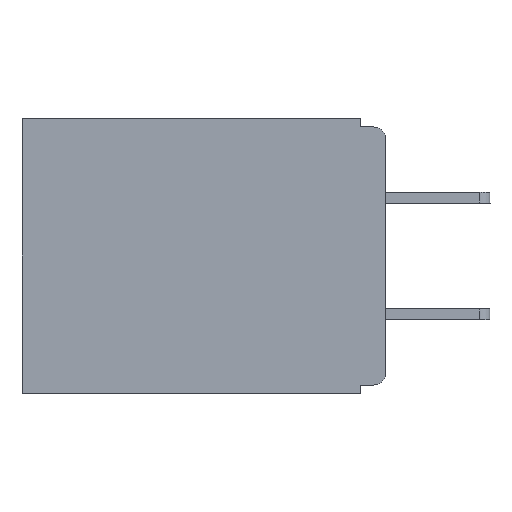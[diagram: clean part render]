
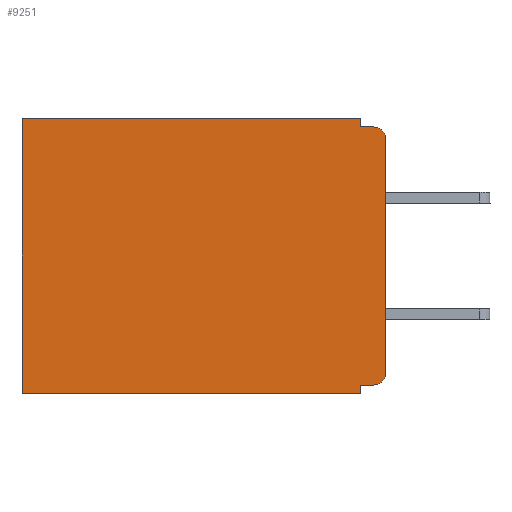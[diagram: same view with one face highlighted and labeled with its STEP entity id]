
A CAD part, left-side view. The second image highlights one B-rep face of the part: STEP entity #9251.
In plain terms, the highlighted planar face has unit normal (-1, 0, 0).
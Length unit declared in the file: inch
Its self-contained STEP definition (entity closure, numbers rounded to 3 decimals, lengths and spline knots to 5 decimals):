
#112 = CARTESIAN_POINT ( 'NONE',  ( 0.3, 0., -0.33 ) ) ;
#113 = ORIENTED_EDGE ( 'NONE', *, *, #10455, .T. ) ;
#322 = VECTOR ( 'NONE', #4174, 39.37008 ) ;
#392 = VERTEX_POINT ( 'NONE', #700 ) ;
#411 = ORIENTED_EDGE ( 'NONE', *, *, #10589, .T. ) ;
#700 = CARTESIAN_POINT ( 'NONE',  ( 0.3, 0.031, -0.01 ) ) ;
#881 = DIRECTION ( 'NONE',  ( 0., 0., -1. ) ) ;
#925 = VECTOR ( 'NONE', #10698, 39.37008 ) ;
#952 = LINE ( 'NONE', #10044, #9979 ) ;
#1090 = EDGE_CURVE ( 'NONE', #5036, #7505, #2635, .T. ) ;
#1230 = EDGE_CURVE ( 'NONE', #2956, #392, #1493, .T. ) ;
#1237 = VECTOR ( 'NONE', #881, 39.37008 ) ;
#1493 = LINE ( 'NONE', #9932, #1237 ) ;
#1507 = EDGE_LOOP ( 'NONE', ( #8773, #411, #9183, #10623, #9588, #2218, #10093, #7792, #8123, #113 ) ) ;
#1562 = DIRECTION ( 'NONE',  ( 0., 0., -1. ) ) ;
#1647 = CIRCLE ( 'NONE', #2615, 0.015 ) ;
#1676 = EDGE_CURVE ( 'NONE', #10653, #7437, #5539, .T. ) ;
#1992 = EDGE_CURVE ( 'NONE', #2956, #8823, #952, .T. ) ;
#2188 = VECTOR ( 'NONE', #4564, 39.37008 ) ;
#2218 = ORIENTED_EDGE ( 'NONE', *, *, #5886, .T. ) ;
#2301 = DIRECTION ( 'NONE',  ( -1., 0., 0. ) ) ;
#2525 = DIRECTION ( 'NONE',  ( 0., 0., -1. ) ) ;
#2615 = AXIS2_PLACEMENT_3D ( 'NONE', #8127, #2301, #7282 ) ;
#2635 = LINE ( 'NONE', #8255, #322 ) ;
#2956 = VERTEX_POINT ( 'NONE', #6523 ) ;
#3293 = EDGE_CURVE ( 'NONE', #392, #8702, #8289, .T. ) ;
#3481 = VERTEX_POINT ( 'NONE', #6968 ) ;
#3605 = VERTEX_POINT ( 'NONE', #6253 ) ;
#3878 = CARTESIAN_POINT ( 'NONE',  ( 0.3, 0.031, -0.33 ) ) ;
#4119 = DIRECTION ( 'NONE',  ( 0., 1., 0. ) ) ;
#4156 = EDGE_CURVE ( 'NONE', #7437, #3481, #9274, .T. ) ;
#4174 = DIRECTION ( 'NONE',  ( 0., 0., -1. ) ) ;
#4404 = CARTESIAN_POINT ( 'NONE',  ( 0.3, 0.437, 0. ) ) ;
#4564 = DIRECTION ( 'NONE',  ( 0., 1., 0. ) ) ;
#4778 = CARTESIAN_POINT ( 'NONE',  ( 0.3, 0., -0.025 ) ) ;
#4897 = VECTOR ( 'NONE', #4119, 39.37008 ) ;
#5036 = VERTEX_POINT ( 'NONE', #4778 ) ;
#5539 = LINE ( 'NONE', #3878, #9664 ) ;
#5593 = AXIS2_PLACEMENT_3D ( 'NONE', #9767, #8970, #1562 ) ;
#5886 = EDGE_CURVE ( 'NONE', #8823, #3481, #10051, .T. ) ;
#6253 = CARTESIAN_POINT ( 'NONE',  ( 0.3, 0.015, -0.32 ) ) ;
#6406 = DIRECTION ( 'NONE',  ( 0., 0., -1. ) ) ;
#6487 = LINE ( 'NONE', #8383, #4897 ) ;
#6523 = CARTESIAN_POINT ( 'NONE',  ( 0.3, 0.031, 0. ) ) ;
#6708 = PLANE ( 'NONE',  #6716 ) ;
#6716 = AXIS2_PLACEMENT_3D ( 'NONE', #112, #9090, #2525 ) ;
#6800 = DIRECTION ( 'NONE',  ( 0., 1., 0. ) ) ;
#6950 = CARTESIAN_POINT ( 'NONE',  ( 0.3, 0., -0.305 ) ) ;
#6968 = CARTESIAN_POINT ( 'NONE',  ( 0.3, 0.437, -0.33 ) ) ;
#7282 = DIRECTION ( 'NONE',  ( 0., 0., -1. ) ) ;
#7308 = CARTESIAN_POINT ( 'NONE',  ( 0.3, 0., -0.01 ) ) ;
#7437 = VERTEX_POINT ( 'NONE', #10022 ) ;
#7505 = VERTEX_POINT ( 'NONE', #6950 ) ;
#7650 = FACE_OUTER_BOUND ( 'NONE', #1507, .T. ) ;
#7792 = ORIENTED_EDGE ( 'NONE', *, *, #1676, .F. ) ;
#7889 = VECTOR ( 'NONE', #9708, 39.37008 ) ;
#8123 = ORIENTED_EDGE ( 'NONE', *, *, #8329, .F. ) ;
#8127 = CARTESIAN_POINT ( 'NONE',  ( 0.3, 0.015, -0.025 ) ) ;
#8255 = CARTESIAN_POINT ( 'NONE',  ( 0.3, 0., -0.33 ) ) ;
#8289 = LINE ( 'NONE', #7308, #925 ) ;
#8329 = EDGE_CURVE ( 'NONE', #3605, #10653, #6487, .T. ) ;
#8383 = CARTESIAN_POINT ( 'NONE',  ( 0.3, 0., -0.32 ) ) ;
#8702 = VERTEX_POINT ( 'NONE', #10594 ) ;
#8773 = ORIENTED_EDGE ( 'NONE', *, *, #1090, .F. ) ;
#8823 = VERTEX_POINT ( 'NONE', #4404 ) ;
#8970 = DIRECTION ( 'NONE',  ( -1., 0., 0. ) ) ;
#9090 = DIRECTION ( 'NONE',  ( 1., 0., 0. ) ) ;
#9183 = ORIENTED_EDGE ( 'NONE', *, *, #3293, .F. ) ;
#9251 = ADVANCED_FACE ( 'NONE', ( #7650 ), #6708, .F. ) ;
#9274 = LINE ( 'NONE', #9475, #2188 ) ;
#9475 = CARTESIAN_POINT ( 'NONE',  ( 0.3, 0., -0.33 ) ) ;
#9588 = ORIENTED_EDGE ( 'NONE', *, *, #1992, .T. ) ;
#9664 = VECTOR ( 'NONE', #6406, 39.37008 ) ;
#9708 = DIRECTION ( 'NONE',  ( 0., 0., -1. ) ) ;
#9726 = CARTESIAN_POINT ( 'NONE',  ( 0.3, 0.031, -0.32 ) ) ;
#9767 = CARTESIAN_POINT ( 'NONE',  ( 0.3, 0.015, -0.305 ) ) ;
#9893 = CIRCLE ( 'NONE', #5593, 0.015 ) ;
#9932 = CARTESIAN_POINT ( 'NONE',  ( 0.3, 0.031, 0. ) ) ;
#9979 = VECTOR ( 'NONE', #6800, 39.37008 ) ;
#10022 = CARTESIAN_POINT ( 'NONE',  ( 0.3, 0.031, -0.33 ) ) ;
#10044 = CARTESIAN_POINT ( 'NONE',  ( 0.3, 0., 0. ) ) ;
#10051 = LINE ( 'NONE', #10435, #7889 ) ;
#10093 = ORIENTED_EDGE ( 'NONE', *, *, #4156, .F. ) ;
#10435 = CARTESIAN_POINT ( 'NONE',  ( 0.3, 0.437, -0.33 ) ) ;
#10455 = EDGE_CURVE ( 'NONE', #3605, #7505, #9893, .T. ) ;
#10589 = EDGE_CURVE ( 'NONE', #5036, #8702, #1647, .T. ) ;
#10594 = CARTESIAN_POINT ( 'NONE',  ( 0.3, 0.015, -0.01 ) ) ;
#10623 = ORIENTED_EDGE ( 'NONE', *, *, #1230, .F. ) ;
#10653 = VERTEX_POINT ( 'NONE', #9726 ) ;
#10698 = DIRECTION ( 'NONE',  ( 0., -1., 0. ) ) ;
